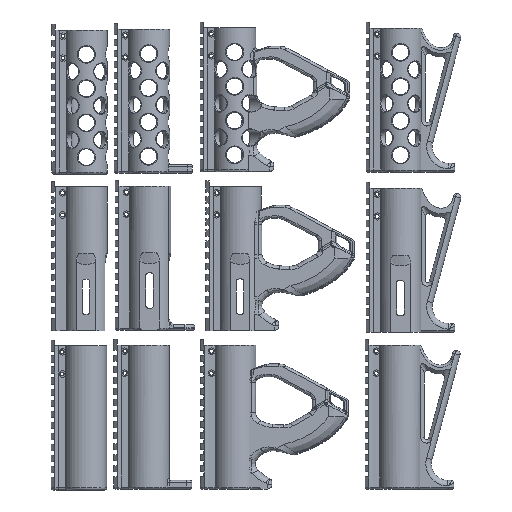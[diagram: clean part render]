
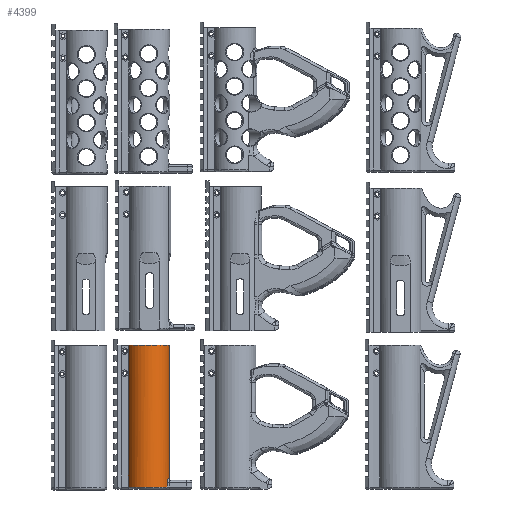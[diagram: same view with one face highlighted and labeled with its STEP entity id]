
A CAD part, left-side view. The second image highlights one B-rep face of the part: STEP entity #4399.
In plain terms, the highlighted cylindrical face has radius 19.2 mm (diameter 38.4 mm), a partial arc.
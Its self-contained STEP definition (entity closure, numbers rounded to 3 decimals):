
#4399=ADVANCED_FACE('',(#7887),#6950,.T.);
#6950=CYLINDRICAL_SURFACE('',#58027,19.2);
#7887=FACE_OUTER_BOUND('',#10830,.T.);
#10830=EDGE_LOOP('',(#29060,#29061,#29062,#29063,#29064,#29065,#29066,#29067,
#29068,#29069));
#13687=B_SPLINE_CURVE_WITH_KNOTS('',3,(#80508,#80509,#80510,#80511,#80512),
 .UNSPECIFIED.,.F.,.F.,(4,1,4),(0.,0.571,1.),.UNSPECIFIED.);
#13688=B_SPLINE_CURVE_WITH_KNOTS('',3,(#80516,#80517,#80518,#80519,#80520,
#80521),.UNSPECIFIED.,.F.,.F.,(4,1,1,4),(0.,0.286,0.571,
1.),.UNSPECIFIED.);
#16706=LINE('',#80498,#21847);
#16707=LINE('',#80502,#21848);
#16708=LINE('',#80506,#21849);
#16709=LINE('',#80523,#21850);
#21847=VECTOR('',#63578,1.);
#21848=VECTOR('',#63581,1.);
#21849=VECTOR('',#63584,1.);
#21850=VECTOR('',#63587,1.);
#29060=ORIENTED_EDGE('',*,*,#49747,.F.);
#29061=ORIENTED_EDGE('',*,*,#49748,.T.);
#29062=ORIENTED_EDGE('',*,*,#49749,.F.);
#29063=ORIENTED_EDGE('',*,*,#49750,.T.);
#29064=ORIENTED_EDGE('',*,*,#49751,.F.);
#29065=ORIENTED_EDGE('',*,*,#49752,.F.);
#29066=ORIENTED_EDGE('',*,*,#49753,.F.);
#29067=ORIENTED_EDGE('',*,*,#49754,.F.);
#29068=ORIENTED_EDGE('',*,*,#49755,.F.);
#29069=ORIENTED_EDGE('',*,*,#49756,.F.);
#43826=VERTEX_POINT('',#80496);
#43827=VERTEX_POINT('',#80497);
#43828=VERTEX_POINT('',#80499);
#43829=VERTEX_POINT('',#80501);
#43830=VERTEX_POINT('',#80503);
#43831=VERTEX_POINT('',#80505);
#43832=VERTEX_POINT('',#80507);
#43833=VERTEX_POINT('',#80513);
#43834=VERTEX_POINT('',#80515);
#43835=VERTEX_POINT('',#80522);
#49747=EDGE_CURVE('',#43826,#43827,#56780,.T.);
#49748=EDGE_CURVE('',#43826,#43828,#16706,.T.);
#49749=EDGE_CURVE('',#43829,#43828,#56781,.T.);
#49750=EDGE_CURVE('',#43829,#43830,#16707,.T.);
#49751=EDGE_CURVE('',#43831,#43830,#56782,.T.);
#49752=EDGE_CURVE('',#43832,#43831,#16708,.T.);
#49753=EDGE_CURVE('',#43833,#43832,#13687,.T.);
#49754=EDGE_CURVE('',#43834,#43833,#56783,.T.);
#49755=EDGE_CURVE('',#43835,#43834,#13688,.T.);
#49756=EDGE_CURVE('',#43827,#43835,#16709,.T.);
#56780=CIRCLE('',#58023,19.2);
#56781=CIRCLE('',#58024,19.2);
#56782=CIRCLE('',#58025,19.2);
#56783=CIRCLE('',#58026,19.2);
#58023=AXIS2_PLACEMENT_3D('',#80495,#63576,#63577);
#58024=AXIS2_PLACEMENT_3D('',#80500,#63579,#63580);
#58025=AXIS2_PLACEMENT_3D('',#80504,#63582,#63583);
#58026=AXIS2_PLACEMENT_3D('',#80514,#63585,#63586);
#58027=AXIS2_PLACEMENT_3D('',#80524,#63588,#63589);
#63576=DIRECTION('',(0.,0.,-1.));
#63577=DIRECTION('',(1.,0.008,0.));
#63578=DIRECTION('',(0.,0.,1.));
#63579=DIRECTION('',(0.,0.,1.));
#63580=DIRECTION('',(1.,0.,0.));
#63581=DIRECTION('',(0.,0.,-1.));
#63582=DIRECTION('',(0.,0.,-1.));
#63583=DIRECTION('',(-1.,0.008,0.));
#63584=DIRECTION('',(0.,0.,-1.));
#63585=DIRECTION('',(0.,0.,-1.));
#63586=DIRECTION('',(0.,-1.,0.));
#63587=DIRECTION('',(0.,0.,1.));
#63588=DIRECTION('',(0.,0.,-1.));
#63589=DIRECTION('',(0.,-1.,0.));
#80495=CARTESIAN_POINT('',(0.,-1.622,-343.977));
#80496=CARTESIAN_POINT('',(7.2,16.177,-343.977));
#80497=CARTESIAN_POINT('',(8.604,-18.786,-343.977));
#80498=CARTESIAN_POINT('',(7.2,16.177,-216.977));
#80499=CARTESIAN_POINT('',(7.2,16.177,-215.477));
#80500=CARTESIAN_POINT('',(0.,-1.622,-215.477));
#80501=CARTESIAN_POINT('',(-7.2,16.177,-215.477));
#80502=CARTESIAN_POINT('',(-7.2,16.177,-238.977));
#80503=CARTESIAN_POINT('',(-7.2,16.177,-343.977));
#80504=CARTESIAN_POINT('',(0.,-1.622,-343.977));
#80505=CARTESIAN_POINT('',(-8.604,-18.786,-343.977));
#80506=CARTESIAN_POINT('',(-8.604,-18.786,-238.977));
#80507=CARTESIAN_POINT('',(-8.604,-18.786,-339.977));
#80508=CARTESIAN_POINT('',(-4.981,-20.164,-335.977));
#80509=CARTESIAN_POINT('',(-6.063,-19.874,-335.977));
#80510=CARTESIAN_POINT('',(-7.886,-19.17,-336.932));
#80511=CARTESIAN_POINT('',(-8.604,-18.786,-339.049));
#80512=CARTESIAN_POINT('',(-8.604,-18.786,-339.977));
#80513=CARTESIAN_POINT('',(-4.981,-20.164,-335.977));
#80514=CARTESIAN_POINT('',(0.,-1.622,-335.977));
#80515=CARTESIAN_POINT('',(4.981,-20.164,-335.977));
#80516=CARTESIAN_POINT('',(8.604,-18.786,-339.977));
#80517=CARTESIAN_POINT('',(8.604,-18.786,-339.358));
#80518=CARTESIAN_POINT('',(8.333,-18.924,-338.128));
#80519=CARTESIAN_POINT('',(7.108,-19.486,-336.486));
#80520=CARTESIAN_POINT('',(5.792,-19.947,-335.977));
#80521=CARTESIAN_POINT('',(4.981,-20.164,-335.977));
#80522=CARTESIAN_POINT('',(8.604,-18.786,-339.977));
#80523=CARTESIAN_POINT('',(8.604,-18.786,-238.977));
#80524=CARTESIAN_POINT('',(0.,-1.622,-238.977));
